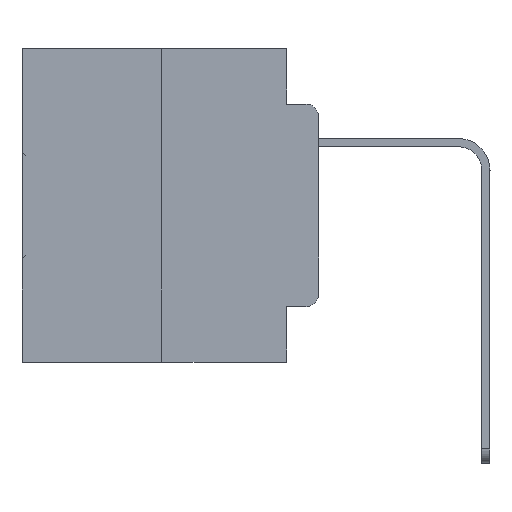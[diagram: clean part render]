
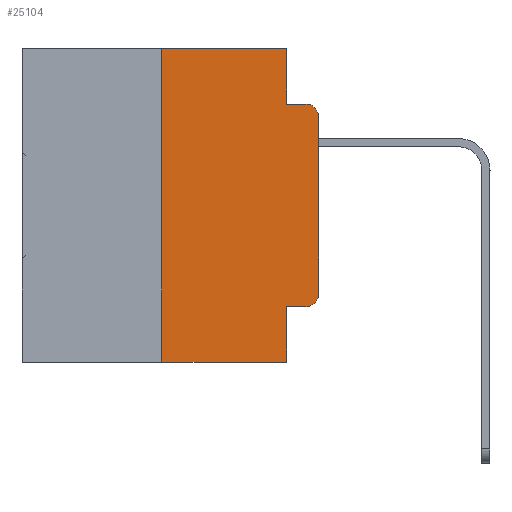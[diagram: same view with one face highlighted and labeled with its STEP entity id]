
A CAD part, left-side view. The second image highlights one B-rep face of the part: STEP entity #25104.
In plain terms, the highlighted planar face has unit normal (-1, 0, 0).
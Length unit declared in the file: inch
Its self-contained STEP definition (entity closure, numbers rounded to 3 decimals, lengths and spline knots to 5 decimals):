
#347 = ORIENTED_EDGE ( 'NONE', *, *, #25997, .F. ) ;
#394 = LINE ( 'NONE', #11602, #5875 ) ;
#1311 = CARTESIAN_POINT ( 'NONE',  ( 0., 0.051, -0.4115 ) ) ;
#2084 = VECTOR ( 'NONE', #6343, 39.37008 ) ;
#2184 = CARTESIAN_POINT ( 'NONE',  ( 0., 0.02, -0.0885 ) ) ;
#3112 = EDGE_CURVE ( 'NONE', #22406, #14775, #20280, .T. ) ;
#3494 = CARTESIAN_POINT ( 'NONE',  ( 0., 0.051, -0.0885 ) ) ;
#3634 = LINE ( 'NONE', #10274, #27723 ) ;
#3712 = AXIS2_PLACEMENT_3D ( 'NONE', #5455, #22086, #12590 ) ;
#4075 = ORIENTED_EDGE ( 'NONE', *, *, #24731, .F. ) ;
#4574 = VERTEX_POINT ( 'NONE', #4610 ) ;
#4610 = CARTESIAN_POINT ( 'NONE',  ( 0., 0.02, -0.4115 ) ) ;
#5029 = CARTESIAN_POINT ( 'NONE',  ( 0., 0.051, -0.4115 ) ) ;
#5455 = CARTESIAN_POINT ( 'NONE',  ( 0., 0.02, -0.1085 ) ) ;
#5875 = VECTOR ( 'NONE', #14136, 39.37008 ) ;
#5922 = EDGE_CURVE ( 'NONE', #4574, #22406, #17288, .T. ) ;
#6101 = CARTESIAN_POINT ( 'NONE',  ( 0., 0.051, 0. ) ) ;
#6343 = DIRECTION ( 'NONE',  ( 0., 0., -1. ) ) ;
#6369 = CARTESIAN_POINT ( 'NONE',  ( 0., 0.051, -0.5 ) ) ;
#6537 = EDGE_CURVE ( 'NONE', #11424, #4574, #9668, .T. ) ;
#6651 = CARTESIAN_POINT ( 'NONE',  ( 0., 0.051, -0.0885 ) ) ;
#6659 = ORIENTED_EDGE ( 'NONE', *, *, #6537, .T. ) ;
#7743 = EDGE_CURVE ( 'NONE', #29729, #11377, #24927, .T. ) ;
#8202 = VECTOR ( 'NONE', #15559, 39.37008 ) ;
#8221 = VERTEX_POINT ( 'NONE', #27213 ) ;
#8435 = DIRECTION ( 'NONE',  ( 0., 0., -1. ) ) ;
#8472 = CARTESIAN_POINT ( 'NONE',  ( 0., 0.02, -0.3915 ) ) ;
#9123 = DIRECTION ( 'NONE',  ( 1., 0., 0. ) ) ;
#9450 = EDGE_CURVE ( 'NONE', #8221, #29711, #394, .T. ) ;
#9668 = LINE ( 'NONE', #1311, #8202 ) ;
#9812 = CARTESIAN_POINT ( 'NONE',  ( 0., 0.051, 0. ) ) ;
#10274 = CARTESIAN_POINT ( 'NONE',  ( 0., 0.25, 0. ) ) ;
#10905 = DIRECTION ( 'NONE',  ( -1., 0., 0. ) ) ;
#11364 = DIRECTION ( 'NONE',  ( 0., 0., -1. ) ) ;
#11377 = VERTEX_POINT ( 'NONE', #2184 ) ;
#11424 = VERTEX_POINT ( 'NONE', #5029 ) ;
#11602 = CARTESIAN_POINT ( 'NONE',  ( 0., 0.473, -0.5 ) ) ;
#12590 = DIRECTION ( 'NONE',  ( 0., 0., -1. ) ) ;
#12836 = DIRECTION ( 'NONE',  ( 0., -1., 0. ) ) ;
#12871 = EDGE_CURVE ( 'NONE', #14775, #11377, #16883, .T. ) ;
#13155 = CARTESIAN_POINT ( 'NONE',  ( 0., 0.051, 0. ) ) ;
#13248 = DIRECTION ( 'NONE',  ( 0., 0., -1. ) ) ;
#13451 = ORIENTED_EDGE ( 'NONE', *, *, #3112, .T. ) ;
#13856 = ORIENTED_EDGE ( 'NONE', *, *, #7743, .F. ) ;
#13884 = LINE ( 'NONE', #14210, #24870 ) ;
#14136 = DIRECTION ( 'NONE',  ( 0., -1., 0. ) ) ;
#14210 = CARTESIAN_POINT ( 'NONE',  ( 0., 0.473, 0. ) ) ;
#14775 = VERTEX_POINT ( 'NONE', #27628 ) ;
#14925 = ORIENTED_EDGE ( 'NONE', *, *, #21692, .F. ) ;
#15354 = ORIENTED_EDGE ( 'NONE', *, *, #12871, .T. ) ;
#15559 = DIRECTION ( 'NONE',  ( 0., -1., 0. ) ) ;
#15629 = VERTEX_POINT ( 'NONE', #21528 ) ;
#15664 = AXIS2_PLACEMENT_3D ( 'NONE', #28008, #9123, #11364 ) ;
#16268 = LINE ( 'NONE', #13155, #2084 ) ;
#16883 = CIRCLE ( 'NONE', #3712, 0.02 ) ;
#17203 = EDGE_LOOP ( 'NONE', ( #13451, #15354, #13856, #347, #14925, #4075, #28137, #22961, #6659, #20072 ) ) ;
#17288 = CIRCLE ( 'NONE', #22260, 0.02 ) ;
#17551 = CARTESIAN_POINT ( 'NONE',  ( 0., 0., -0.3915 ) ) ;
#17808 = FACE_OUTER_BOUND ( 'NONE', #17203, .T. ) ;
#18670 = VECTOR ( 'NONE', #12836, 39.37008 ) ;
#19229 = LINE ( 'NONE', #6101, #25453 ) ;
#19443 = DIRECTION ( 'NONE',  ( 0., 0., 1. ) ) ;
#19537 = VERTEX_POINT ( 'NONE', #9812 ) ;
#19984 = DIRECTION ( 'NONE',  ( 0., 0., 1. ) ) ;
#20072 = ORIENTED_EDGE ( 'NONE', *, *, #5922, .T. ) ;
#20280 = LINE ( 'NONE', #26964, #25424 ) ;
#21528 = CARTESIAN_POINT ( 'NONE',  ( 0., 0.25, 0. ) ) ;
#21692 = EDGE_CURVE ( 'NONE', #15629, #19537, #13884, .T. ) ;
#22086 = DIRECTION ( 'NONE',  ( -1., 0., 0. ) ) ;
#22260 = AXIS2_PLACEMENT_3D ( 'NONE', #8472, #10905, #13248 ) ;
#22406 = VERTEX_POINT ( 'NONE', #17551 ) ;
#22961 = ORIENTED_EDGE ( 'NONE', *, *, #23410, .F. ) ;
#23410 = EDGE_CURVE ( 'NONE', #11424, #29711, #19229, .T. ) ;
#24731 = EDGE_CURVE ( 'NONE', #8221, #15629, #3634, .T. ) ;
#24870 = VECTOR ( 'NONE', #28118, 39.37008 ) ;
#24927 = LINE ( 'NONE', #3494, #18670 ) ;
#25104 = ADVANCED_FACE ( 'NONE', ( #17808 ), #25655, .F. ) ;
#25424 = VECTOR ( 'NONE', #19984, 39.37008 ) ;
#25453 = VECTOR ( 'NONE', #8435, 39.37008 ) ;
#25655 = PLANE ( 'NONE',  #15664 ) ;
#25997 = EDGE_CURVE ( 'NONE', #19537, #29729, #16268, .T. ) ;
#26964 = CARTESIAN_POINT ( 'NONE',  ( 0., 0., 0. ) ) ;
#27213 = CARTESIAN_POINT ( 'NONE',  ( 0., 0.25, -0.5 ) ) ;
#27628 = CARTESIAN_POINT ( 'NONE',  ( 0., 0., -0.1085 ) ) ;
#27723 = VECTOR ( 'NONE', #19443, 39.37008 ) ;
#28008 = CARTESIAN_POINT ( 'NONE',  ( 0., 0.473, 0. ) ) ;
#28118 = DIRECTION ( 'NONE',  ( 0., -1., 0. ) ) ;
#28137 = ORIENTED_EDGE ( 'NONE', *, *, #9450, .T. ) ;
#29711 = VERTEX_POINT ( 'NONE', #6369 ) ;
#29729 = VERTEX_POINT ( 'NONE', #6651 ) ;
